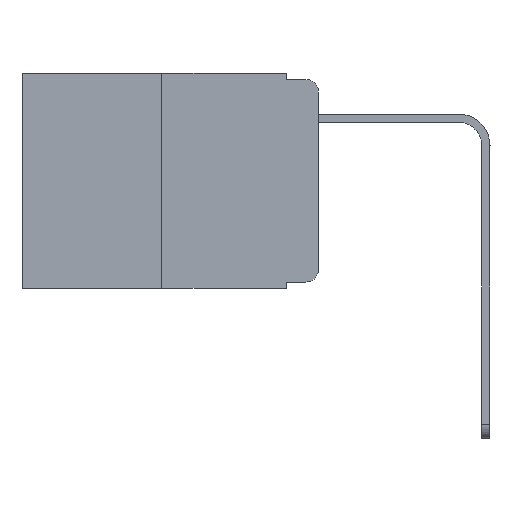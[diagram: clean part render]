
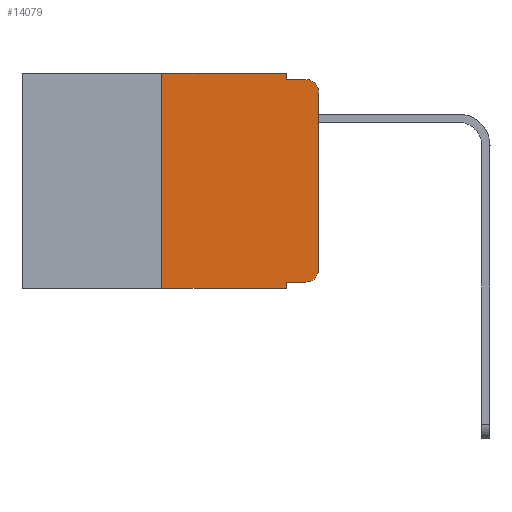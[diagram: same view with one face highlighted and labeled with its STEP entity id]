
A CAD part, left-side view. The second image highlights one B-rep face of the part: STEP entity #14079.
In plain terms, the highlighted planar face has unit normal (-1, 0, 0).
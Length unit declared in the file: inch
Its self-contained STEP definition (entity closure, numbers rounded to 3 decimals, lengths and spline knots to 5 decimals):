
#96 = CARTESIAN_POINT ( 'NONE',  ( 0., 0.25, 0. ) ) ;
#158 = DIRECTION ( 'NONE',  ( 0., 0., -1. ) ) ;
#291 = LINE ( 'NONE', #3852, #14667 ) ;
#645 = ORIENTED_EDGE ( 'NONE', *, *, #14396, .F. ) ;
#717 = LINE ( 'NONE', #5452, #16334 ) ;
#1005 = AXIS2_PLACEMENT_3D ( 'NONE', #1319, #7821, #158 ) ;
#1319 = CARTESIAN_POINT ( 'NONE',  ( 0., 0.02, -0.313 ) ) ;
#1409 = CARTESIAN_POINT ( 'NONE',  ( 0., 0., -0.313 ) ) ;
#1858 = VERTEX_POINT ( 'NONE', #7925 ) ;
#1928 = EDGE_CURVE ( 'NONE', #14051, #4774, #4682, .T. ) ;
#2526 = ORIENTED_EDGE ( 'NONE', *, *, #7523, .F. ) ;
#2614 = ORIENTED_EDGE ( 'NONE', *, *, #16776, .F. ) ;
#2709 = DIRECTION ( 'NONE',  ( -1., 0., 0. ) ) ;
#2929 = CARTESIAN_POINT ( 'NONE',  ( 0., 0.02, -0.03 ) ) ;
#3319 = CARTESIAN_POINT ( 'NONE',  ( 0., 0.051, 0. ) ) ;
#3342 = LINE ( 'NONE', #11107, #9112 ) ;
#3350 = ORIENTED_EDGE ( 'NONE', *, *, #1928, .F. ) ;
#3468 = CIRCLE ( 'NONE', #4560, 0.02 ) ;
#3486 = CARTESIAN_POINT ( 'NONE',  ( 0., 0.02, -0.333 ) ) ;
#3519 = FACE_OUTER_BOUND ( 'NONE', #11335, .T. ) ;
#3852 = CARTESIAN_POINT ( 'NONE',  ( 0., 0.473, -0.343 ) ) ;
#4078 = DIRECTION ( 'NONE',  ( 0., 0., -1. ) ) ;
#4328 = CARTESIAN_POINT ( 'NONE',  ( 0., 0.051, -0.343 ) ) ;
#4339 = EDGE_CURVE ( 'NONE', #4573, #12919, #7915, .T. ) ;
#4560 = AXIS2_PLACEMENT_3D ( 'NONE', #2929, #2709, #15837 ) ;
#4573 = VERTEX_POINT ( 'NONE', #3486 ) ;
#4682 = LINE ( 'NONE', #96, #11282 ) ;
#4739 = VECTOR ( 'NONE', #13154, 39.37008 ) ;
#4774 = VERTEX_POINT ( 'NONE', #8573 ) ;
#4941 = CARTESIAN_POINT ( 'NONE',  ( 0., 0.25, -0.343 ) ) ;
#5080 = VECTOR ( 'NONE', #9254, 39.37008 ) ;
#5092 = VERTEX_POINT ( 'NONE', #13584 ) ;
#5396 = EDGE_CURVE ( 'NONE', #12919, #12724, #3342, .T. ) ;
#5452 = CARTESIAN_POINT ( 'NONE',  ( 0., 0.051, -0.01 ) ) ;
#5458 = ORIENTED_EDGE ( 'NONE', *, *, #16079, .T. ) ;
#6733 = DIRECTION ( 'NONE',  ( 0., -1., 0. ) ) ;
#6812 = ORIENTED_EDGE ( 'NONE', *, *, #5396, .T. ) ;
#7162 = VERTEX_POINT ( 'NONE', #7410 ) ;
#7410 = CARTESIAN_POINT ( 'NONE',  ( 0., 0.051, 0. ) ) ;
#7523 = EDGE_CURVE ( 'NONE', #4774, #7162, #15419, .T. ) ;
#7821 = DIRECTION ( 'NONE',  ( -1., 0., 0. ) ) ;
#7846 = CARTESIAN_POINT ( 'NONE',  ( 0., 0.051, -0.333 ) ) ;
#7909 = CARTESIAN_POINT ( 'NONE',  ( 0., 0.051, 0. ) ) ;
#7915 = CIRCLE ( 'NONE', #1005, 0.02 ) ;
#7925 = CARTESIAN_POINT ( 'NONE',  ( 0., 0.02, -0.01 ) ) ;
#8294 = AXIS2_PLACEMENT_3D ( 'NONE', #11797, #10653, #4078 ) ;
#8513 = DIRECTION ( 'NONE',  ( 0., 0., 1. ) ) ;
#8573 = CARTESIAN_POINT ( 'NONE',  ( 0., 0.25, 0. ) ) ;
#9112 = VECTOR ( 'NONE', #8513, 39.37008 ) ;
#9254 = DIRECTION ( 'NONE',  ( 0., 0., -1. ) ) ;
#9889 = LINE ( 'NONE', #3319, #13971 ) ;
#9935 = DIRECTION ( 'NONE',  ( 0., 0., -1. ) ) ;
#10604 = CARTESIAN_POINT ( 'NONE',  ( 0., 0.051, -0.333 ) ) ;
#10653 = DIRECTION ( 'NONE',  ( 1., 0., 0. ) ) ;
#11071 = EDGE_CURVE ( 'NONE', #14051, #13170, #291, .T. ) ;
#11107 = CARTESIAN_POINT ( 'NONE',  ( 0., 0., 0. ) ) ;
#11282 = VECTOR ( 'NONE', #14436, 39.37008 ) ;
#11335 = EDGE_LOOP ( 'NONE', ( #6812, #16520, #16797, #2614, #2526, #3350, #11813, #645, #5458, #14100 ) ) ;
#11797 = CARTESIAN_POINT ( 'NONE',  ( 0., 0.473, 0. ) ) ;
#11813 = ORIENTED_EDGE ( 'NONE', *, *, #11071, .T. ) ;
#11922 = EDGE_CURVE ( 'NONE', #5092, #1858, #717, .T. ) ;
#11969 = PLANE ( 'NONE',  #8294 ) ;
#12033 = DIRECTION ( 'NONE',  ( 0., -1., 0. ) ) ;
#12724 = VERTEX_POINT ( 'NONE', #12862 ) ;
#12862 = CARTESIAN_POINT ( 'NONE',  ( 0., 0., -0.03 ) ) ;
#12919 = VERTEX_POINT ( 'NONE', #1409 ) ;
#13001 = VERTEX_POINT ( 'NONE', #7846 ) ;
#13154 = DIRECTION ( 'NONE',  ( 0., -1., 0. ) ) ;
#13170 = VERTEX_POINT ( 'NONE', #4328 ) ;
#13584 = CARTESIAN_POINT ( 'NONE',  ( 0., 0.051, -0.01 ) ) ;
#13971 = VECTOR ( 'NONE', #9935, 39.37008 ) ;
#14051 = VERTEX_POINT ( 'NONE', #4941 ) ;
#14079 = ADVANCED_FACE ( 'NONE', ( #3519 ), #11969, .F. ) ;
#14100 = ORIENTED_EDGE ( 'NONE', *, *, #4339, .T. ) ;
#14396 = EDGE_CURVE ( 'NONE', #13001, #13170, #9889, .T. ) ;
#14436 = DIRECTION ( 'NONE',  ( 0., 0., 1. ) ) ;
#14507 = VECTOR ( 'NONE', #12033, 39.37008 ) ;
#14667 = VECTOR ( 'NONE', #15537, 39.37008 ) ;
#15144 = LINE ( 'NONE', #7909, #5080 ) ;
#15419 = LINE ( 'NONE', #15653, #4739 ) ;
#15480 = EDGE_CURVE ( 'NONE', #12724, #1858, #3468, .T. ) ;
#15537 = DIRECTION ( 'NONE',  ( 0., -1., 0. ) ) ;
#15540 = LINE ( 'NONE', #10604, #14507 ) ;
#15653 = CARTESIAN_POINT ( 'NONE',  ( 0., 0.473, 0. ) ) ;
#15837 = DIRECTION ( 'NONE',  ( 0., 0., -1. ) ) ;
#16079 = EDGE_CURVE ( 'NONE', #13001, #4573, #15540, .T. ) ;
#16334 = VECTOR ( 'NONE', #6733, 39.37008 ) ;
#16520 = ORIENTED_EDGE ( 'NONE', *, *, #15480, .T. ) ;
#16776 = EDGE_CURVE ( 'NONE', #7162, #5092, #15144, .T. ) ;
#16797 = ORIENTED_EDGE ( 'NONE', *, *, #11922, .F. ) ;
